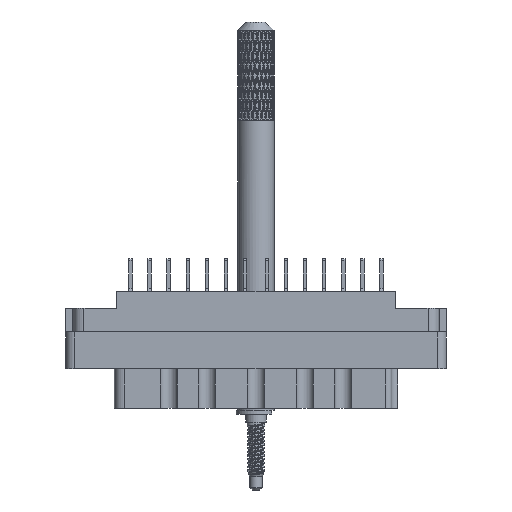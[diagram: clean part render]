
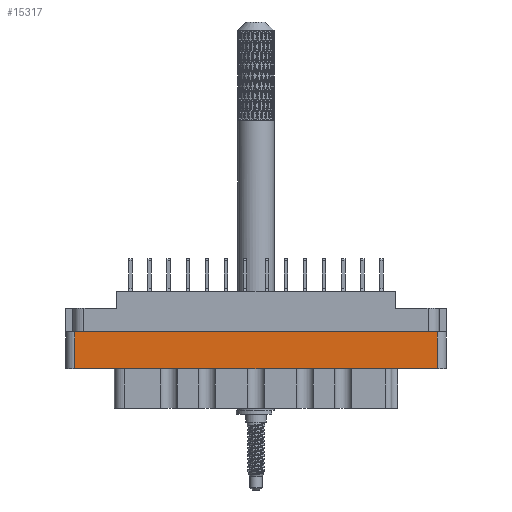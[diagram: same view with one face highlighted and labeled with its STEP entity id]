
A CAD part, front view. The second image highlights one B-rep face of the part: STEP entity #15317.
In plain terms, the highlighted planar face has unit normal (0, -1, 0).
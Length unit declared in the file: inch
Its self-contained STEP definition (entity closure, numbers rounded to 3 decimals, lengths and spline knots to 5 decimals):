
#2710 = PLANE ( 'NONE',  #39468 ) ;
#3041 = DIRECTION ( 'NONE',  ( -1., 0., 0. ) ) ;
#3119 = VERTEX_POINT ( 'NONE', #20539 ) ;
#3411 = ORIENTED_EDGE ( 'NONE', *, *, #60213, .F. ) ;
#8484 = VECTOR ( 'NONE', #71628, 39.37008 ) ;
#11764 = CARTESIAN_POINT ( 'NONE',  ( 0., -0.438, -0.529 ) ) ;
#15317 = ADVANCED_FACE ( 'NONE', ( #100371 ), #2710, .T. ) ;
#17194 = VECTOR ( 'NONE', #44220, 39.37008 ) ;
#20539 = CARTESIAN_POINT ( 'NONE',  ( -1.234, -0.438, -0.529 ) ) ;
#21564 = DIRECTION ( 'NONE',  ( 0., -1., 0. ) ) ;
#24423 = EDGE_LOOP ( 'NONE', ( #85337, #35855, #3411, #79714 ) ) ;
#24744 = VERTEX_POINT ( 'NONE', #71282 ) ;
#28122 = VECTOR ( 'NONE', #102421, 39.37008 ) ;
#35107 = CARTESIAN_POINT ( 'NONE',  ( 0., -0.438, -0.277 ) ) ;
#35855 = ORIENTED_EDGE ( 'NONE', *, *, #79294, .T. ) ;
#38267 = LINE ( 'NONE', #35107, #17194 ) ;
#38737 = VERTEX_POINT ( 'NONE', #58672 ) ;
#39468 = AXIS2_PLACEMENT_3D ( 'NONE', #102378, #21564, #57456 ) ;
#44220 = DIRECTION ( 'NONE',  ( 1., 0., 0. ) ) ;
#56740 = VERTEX_POINT ( 'NONE', #67525 ) ;
#57456 = DIRECTION ( 'NONE',  ( 0., 0., -1. ) ) ;
#58672 = CARTESIAN_POINT ( 'NONE',  ( 1.234, -0.438, -0.529 ) ) ;
#60213 = EDGE_CURVE ( 'NONE', #38737, #3119, #115283, .T. ) ;
#64792 = LINE ( 'NONE', #92636, #28122 ) ;
#64817 = EDGE_CURVE ( 'NONE', #24744, #56740, #38267, .T. ) ;
#67525 = CARTESIAN_POINT ( 'NONE',  ( 1.234, -0.438, -0.277 ) ) ;
#70853 = CARTESIAN_POINT ( 'NONE',  ( 1.234, -0.438, -0.798 ) ) ;
#71282 = CARTESIAN_POINT ( 'NONE',  ( -1.234, -0.438, -0.277 ) ) ;
#71628 = DIRECTION ( 'NONE',  ( 0., 0., 1. ) ) ;
#79294 = EDGE_CURVE ( 'NONE', #24744, #3119, #64792, .T. ) ;
#79714 = ORIENTED_EDGE ( 'NONE', *, *, #104131, .T. ) ;
#85337 = ORIENTED_EDGE ( 'NONE', *, *, #64817, .F. ) ;
#92636 = CARTESIAN_POINT ( 'NONE',  ( -1.234, -0.438, -0.798 ) ) ;
#100371 = FACE_OUTER_BOUND ( 'NONE', #24423, .T. ) ;
#102378 = CARTESIAN_POINT ( 'NONE',  ( -1.296, -0.438, -0.798 ) ) ;
#102421 = DIRECTION ( 'NONE',  ( 0., 0., -1. ) ) ;
#104131 = EDGE_CURVE ( 'NONE', #38737, #56740, #107208, .T. ) ;
#107208 = LINE ( 'NONE', #70853, #8484 ) ;
#111034 = VECTOR ( 'NONE', #3041, 39.37008 ) ;
#115283 = LINE ( 'NONE', #11764, #111034 ) ;
